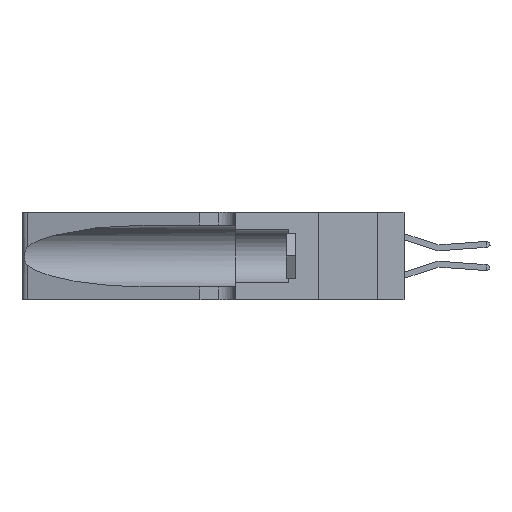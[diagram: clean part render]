
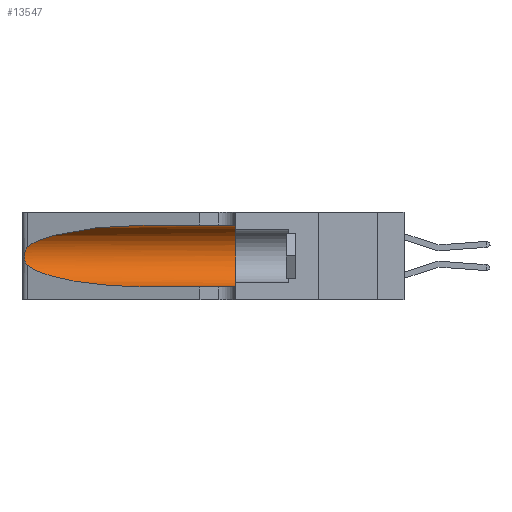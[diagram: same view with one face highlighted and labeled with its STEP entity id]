
A CAD part, left-side view. The second image highlights one B-rep face of the part: STEP entity #13547.
In plain terms, the highlighted cylindrical face has radius 3.308 mm (diameter 6.617 mm), a partial arc.
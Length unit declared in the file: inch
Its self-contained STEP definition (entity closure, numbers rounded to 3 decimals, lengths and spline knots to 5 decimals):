
#613 = CARTESIAN_POINT ( 'NONE',  ( 0.25487, 1.22718, 0.14631 ) ) ;
#1164 = CARTESIAN_POINT ( 'NONE',  ( 0.1305, 0.72297, 0.05475 ) ) ;
#1874 = EDGE_CURVE ( 'NONE', #15256, #12339, #36423, .T. ) ;
#2045 = CARTESIAN_POINT ( 'NONE',  ( 0.25856, 1.23593, 0.16098 ) ) ;
#4103 = CYLINDRICAL_SURFACE ( 'NONE', #28926, 0.13025 ) ;
#5245 = CARTESIAN_POINT ( 'NONE',  ( 0.25639, 1.23186, 0.15144 ) ) ;
#5693 = CARTESIAN_POINT ( 'NONE',  ( 0.1305, 0.72297, 0.31525 ) ) ;
#6374 = EDGE_CURVE ( 'NONE', #16977, #22656, #22067, .T. ) ;
#7048 = CARTESIAN_POINT ( 'NONE',  ( 0.25487, 1.22718, 0.22369 ) ) ;
#7844 = DIRECTION ( 'NONE',  ( 0., 0., -1. ) ) ;
#7876 = VECTOR ( 'NONE', #9777, 39.37008 ) ;
#8242 = CARTESIAN_POINT ( 'NONE',  ( 0.25639, 1.23184, 0.21858 ) ) ;
#8373 = CARTESIAN_POINT ( 'NONE',  ( 0.25487, 1.22718, 0.14631 ) ) ;
#9080 = EDGE_CURVE ( 'NONE', #15099, #15256, #15076, .T. ) ;
#9777 = DIRECTION ( 'NONE',  ( 0., -1., 0. ) ) ;
#10298 = ORIENTED_EDGE ( 'NONE', *, *, #31824, .F. ) ;
#11228 = VERTEX_POINT ( 'NONE', #17074 ) ;
#12013 = CARTESIAN_POINT ( 'NONE',  ( 0.1305, 0.35, 0.05475 ) ) ;
#12339 = VERTEX_POINT ( 'NONE', #613 ) ;
#13547 = ADVANCED_FACE ( 'NONE', ( #29642 ), #4103, .F. ) ;
#14453 = CARTESIAN_POINT ( 'NONE',  ( 0.25854, 1.2359, 0.20912 ) ) ;
#14794 = VECTOR ( 'NONE', #38968, 39.37008 ) ;
#14868 = CARTESIAN_POINT ( 'NONE',  ( 0.18966, 0.96281, 0.31525 ) ) ;
#14999 = CARTESIAN_POINT ( 'NONE',  ( 0.25487, 1.22718, 0.22369 ) ) ;
#15048 = ORIENTED_EDGE ( 'NONE', *, *, #19517, .T. ) ;
#15076 =( BOUNDED_CURVE ( )  B_SPLINE_CURVE ( 3, ( #5693, #14868, #33337, #14999 ),
 .UNSPECIFIED., .F., .T. ) 
 B_SPLINE_CURVE_WITH_KNOTS ( ( 4, 4 ),
 ( 1.5708, 2.84003 ),
 .UNSPECIFIED. ) 
 CURVE ( )  GEOMETRIC_REPRESENTATION_ITEM ( )  RATIONAL_B_SPLINE_CURVE ( ( 1., 0.87, 0.87, 1. ) ) 
 REPRESENTATION_ITEM ( '' )  );
#15098 = LINE ( 'NONE', #28191, #7876 ) ;
#15099 = VERTEX_POINT ( 'NONE', #24851 ) ;
#15256 = VERTEX_POINT ( 'NONE', #7048 ) ;
#16803 = AXIS2_PLACEMENT_3D ( 'NONE', #35524, #17232, #38556 ) ;
#16814 = CARTESIAN_POINT ( 'NONE',  ( 0.1305, 0.72297, 0.05475 ) ) ;
#16977 = VERTEX_POINT ( 'NONE', #1164 ) ;
#17074 = CARTESIAN_POINT ( 'NONE',  ( 0.1305, 0.35, 0.31525 ) ) ;
#17168 = DIRECTION ( 'NONE',  ( 0., -1., 0. ) ) ;
#17232 = DIRECTION ( 'NONE',  ( 0., 1., 0. ) ) ;
#17569 = CARTESIAN_POINT ( 'NONE',  ( 0.26075, 1.23896, 0.19203 ) ) ;
#19517 = EDGE_CURVE ( 'NONE', #12339, #16977, #33478, .T. ) ;
#20383 = EDGE_LOOP ( 'NONE', ( #31107, #37982, #15048, #24724, #26606, #10298 ) ) ;
#20665 = CARTESIAN_POINT ( 'NONE',  ( 0.26017, 1.23833, 0.17102 ) ) ;
#21771 = EDGE_CURVE ( 'NONE', #11228, #22656, #30866, .T. ) ;
#22067 = LINE ( 'NONE', #23833, #14794 ) ;
#22656 = VERTEX_POINT ( 'NONE', #12013 ) ;
#23765 = CARTESIAN_POINT ( 'NONE',  ( 0.25789, 1.23486, 0.15765 ) ) ;
#23833 = CARTESIAN_POINT ( 'NONE',  ( 0.1305, 1.61858, 0.05475 ) ) ;
#24724 = ORIENTED_EDGE ( 'NONE', *, *, #6374, .T. ) ;
#24851 = CARTESIAN_POINT ( 'NONE',  ( 0.1305, 0.72297, 0.31525 ) ) ;
#25928 = CARTESIAN_POINT ( 'NONE',  ( 0.2373, 1.15595, 0.08982 ) ) ;
#26606 = ORIENTED_EDGE ( 'NONE', *, *, #21771, .F. ) ;
#26653 = CARTESIAN_POINT ( 'NONE',  ( 0.25487, 1.22718, 0.22369 ) ) ;
#26790 = CARTESIAN_POINT ( 'NONE',  ( 0.25555, 1.22993, 0.14849 ) ) ;
#28191 = CARTESIAN_POINT ( 'NONE',  ( 0.1305, 1.61858, 0.31525 ) ) ;
#28926 = AXIS2_PLACEMENT_3D ( 'NONE', #32388, #17168, #7844 ) ;
#29642 = FACE_OUTER_BOUND ( 'NONE', #20383, .T. ) ;
#29713 = CARTESIAN_POINT ( 'NONE',  ( 0.25555, 1.22994, 0.2215 ) ) ;
#30866 = CIRCLE ( 'NONE', #16803, 0.13025 ) ;
#31107 = ORIENTED_EDGE ( 'NONE', *, *, #9080, .T. ) ;
#31824 = EDGE_CURVE ( 'NONE', #15099, #11228, #15098, .T. ) ;
#32039 = CARTESIAN_POINT ( 'NONE',  ( 0.25487, 1.22718, 0.14631 ) ) ;
#32388 = CARTESIAN_POINT ( 'NONE',  ( 0.1305, 1.61858, 0.185 ) ) ;
#32797 = CARTESIAN_POINT ( 'NONE',  ( 0.25787, 1.23484, 0.2124 ) ) ;
#33337 = CARTESIAN_POINT ( 'NONE',  ( 0.2373, 1.15595, 0.28018 ) ) ;
#33478 =( BOUNDED_CURVE ( )  B_SPLINE_CURVE ( 3, ( #32039, #25928, #35117, #16814 ),
 .UNSPECIFIED., .F., .T. ) 
 B_SPLINE_CURVE_WITH_KNOTS ( ( 4, 4 ),
 ( 3.44316, 4.71239 ),
 .UNSPECIFIED. ) 
 CURVE ( )  GEOMETRIC_REPRESENTATION_ITEM ( )  RATIONAL_B_SPLINE_CURVE ( ( 1., 0.87, 0.87, 1. ) ) 
 REPRESENTATION_ITEM ( '' )  );
#35117 = CARTESIAN_POINT ( 'NONE',  ( 0.18966, 0.96281, 0.05475 ) ) ;
#35524 = CARTESIAN_POINT ( 'NONE',  ( 0.1305, 0.35, 0.185 ) ) ;
#35861 = CARTESIAN_POINT ( 'NONE',  ( 0.26018, 1.23835, 0.19895 ) ) ;
#36423 = B_SPLINE_CURVE_WITH_KNOTS ( 'NONE', 3,
 ( #26653, #29713, #8242, #32797, #14453, #35861, #17569, #38897, #20665, #2045, #23765, #5245, #26790, #8373 ),
 .UNSPECIFIED., .F., .F.,
 ( 4, 2, 2, 2, 2, 2, 4 ),
 ( 0., 0.00027, 0.00053, 0.00107, 0.0016, 0.00187, 0.00214 ),
 .UNSPECIFIED. ) ;
#37982 = ORIENTED_EDGE ( 'NONE', *, *, #1874, .T. ) ;
#38556 = DIRECTION ( 'NONE',  ( 0., 0., 1. ) ) ;
#38897 = CARTESIAN_POINT ( 'NONE',  ( 0.26075, 1.23896, 0.178 ) ) ;
#38968 = DIRECTION ( 'NONE',  ( 0., -1., 0. ) ) ;
